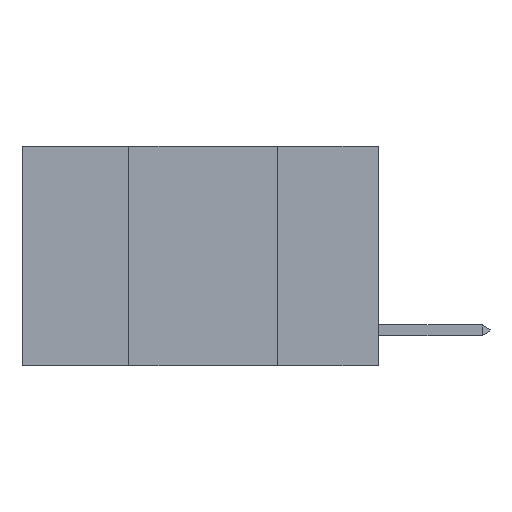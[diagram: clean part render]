
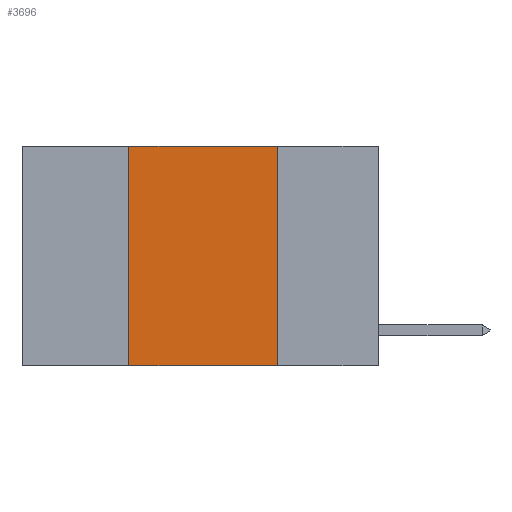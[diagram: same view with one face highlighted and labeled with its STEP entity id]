
A CAD part, left-side view. The second image highlights one B-rep face of the part: STEP entity #3696.
In plain terms, the highlighted planar face has unit normal (-1, 0, 0).
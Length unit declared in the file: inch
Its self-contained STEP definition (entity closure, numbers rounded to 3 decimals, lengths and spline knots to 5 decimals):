
#200 = CARTESIAN_POINT ( 'NONE',  ( 0., 0.6, 0. ) ) ;
#277 = CARTESIAN_POINT ( 'NONE',  ( 0., 0.42, 0. ) ) ;
#440 = CARTESIAN_POINT ( 'NONE',  ( 0., 0.17, 0. ) ) ;
#999 = EDGE_CURVE ( 'NONE', #6595, #9876, #6378, .T. ) ;
#1158 = EDGE_LOOP ( 'NONE', ( #9032, #10157, #4431, #6650 ) ) ;
#1172 = DIRECTION ( 'NONE',  ( 0., 0., -1. ) ) ;
#1304 = CARTESIAN_POINT ( 'NONE',  ( 0., 0.42, -0.37 ) ) ;
#1342 = VECTOR ( 'NONE', #5304, 39.37008 ) ;
#1577 = CARTESIAN_POINT ( 'NONE',  ( 0., 0.17, 0. ) ) ;
#2097 = EDGE_CURVE ( 'NONE', #2405, #9876, #8921, .T. ) ;
#2164 = CARTESIAN_POINT ( 'NONE',  ( 0., 0.42, 0. ) ) ;
#2283 = EDGE_CURVE ( 'NONE', #6595, #10196, #6074, .T. ) ;
#2405 = VERTEX_POINT ( 'NONE', #1577 ) ;
#3519 = DIRECTION ( 'NONE',  ( 1., 0., 0. ) ) ;
#3563 = CARTESIAN_POINT ( 'NONE',  ( 0., 0.6, 0. ) ) ;
#3696 = ADVANCED_FACE ( 'NONE', ( #7433 ), #7381, .F. ) ;
#3712 = AXIS2_PLACEMENT_3D ( 'NONE', #200, #3519, #6639 ) ;
#4431 = ORIENTED_EDGE ( 'NONE', *, *, #2283, .F. ) ;
#4718 = VECTOR ( 'NONE', #8245, 39.37008 ) ;
#5304 = DIRECTION ( 'NONE',  ( 0., 0., 1. ) ) ;
#6074 = LINE ( 'NONE', #2164, #1342 ) ;
#6097 = CARTESIAN_POINT ( 'NONE',  ( 0., 0.17, -0.37 ) ) ;
#6227 = DIRECTION ( 'NONE',  ( 0., -1., 0. ) ) ;
#6378 = LINE ( 'NONE', #9520, #9286 ) ;
#6533 = LINE ( 'NONE', #3563, #4718 ) ;
#6595 = VERTEX_POINT ( 'NONE', #1304 ) ;
#6639 = DIRECTION ( 'NONE',  ( 0., 0., -1. ) ) ;
#6650 = ORIENTED_EDGE ( 'NONE', *, *, #999, .T. ) ;
#7381 = PLANE ( 'NONE',  #3712 ) ;
#7433 = FACE_OUTER_BOUND ( 'NONE', #1158, .T. ) ;
#7753 = EDGE_CURVE ( 'NONE', #10196, #2405, #6533, .T. ) ;
#7816 = VECTOR ( 'NONE', #1172, 39.37008 ) ;
#8245 = DIRECTION ( 'NONE',  ( 0., -1., 0. ) ) ;
#8921 = LINE ( 'NONE', #440, #7816 ) ;
#9032 = ORIENTED_EDGE ( 'NONE', *, *, #2097, .F. ) ;
#9286 = VECTOR ( 'NONE', #6227, 39.37008 ) ;
#9520 = CARTESIAN_POINT ( 'NONE',  ( 0., 0.6, -0.37 ) ) ;
#9876 = VERTEX_POINT ( 'NONE', #6097 ) ;
#10157 = ORIENTED_EDGE ( 'NONE', *, *, #7753, .F. ) ;
#10196 = VERTEX_POINT ( 'NONE', #277 ) ;
